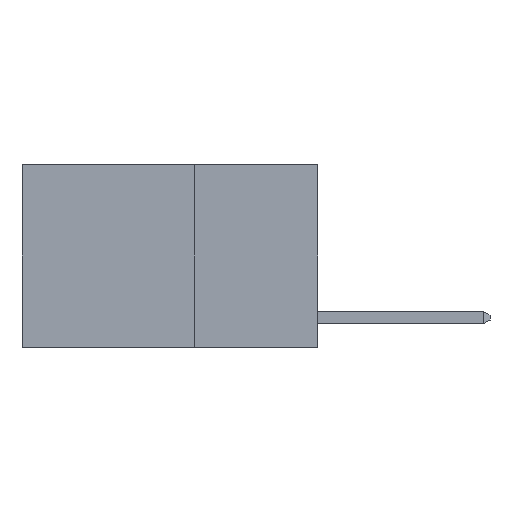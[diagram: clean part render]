
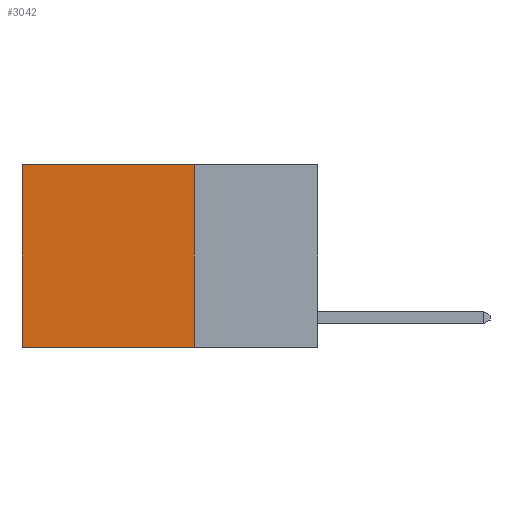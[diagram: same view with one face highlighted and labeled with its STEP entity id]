
A CAD part, left-side view. The second image highlights one B-rep face of the part: STEP entity #3042.
In plain terms, the highlighted planar face has unit normal (-1, 0, 0).
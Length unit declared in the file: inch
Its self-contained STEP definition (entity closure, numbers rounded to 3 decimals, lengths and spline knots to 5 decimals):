
#487 = EDGE_LOOP ( 'NONE', ( #1134, #1333, #1735, #3691 ) ) ;
#552 = CARTESIAN_POINT ( 'NONE',  ( 0.2625, 0.6, 0. ) ) ;
#843 = VECTOR ( 'NONE', #7384, 39.37008 ) ;
#1086 = LINE ( 'NONE', #552, #7396 ) ;
#1132 = VERTEX_POINT ( 'NONE', #3738 ) ;
#1134 = ORIENTED_EDGE ( 'NONE', *, *, #3964, .T. ) ;
#1333 = ORIENTED_EDGE ( 'NONE', *, *, #3685, .F. ) ;
#1570 = VERTEX_POINT ( 'NONE', #8058 ) ;
#1735 = ORIENTED_EDGE ( 'NONE', *, *, #3491, .F. ) ;
#2624 = VECTOR ( 'NONE', #4058, 39.37008 ) ;
#2630 = CARTESIAN_POINT ( 'NONE',  ( 0.2625, 0.25, 0. ) ) ;
#2750 = DIRECTION ( 'NONE',  ( 0., 0., -1. ) ) ;
#3031 = CARTESIAN_POINT ( 'NONE',  ( 0.2625, 0.25, 0. ) ) ;
#3042 = ADVANCED_FACE ( 'NONE', ( #3602 ), #6701, .F. ) ;
#3483 = VECTOR ( 'NONE', #3629, 39.37008 ) ;
#3491 = EDGE_CURVE ( 'NONE', #4470, #3784, #6822, .T. ) ;
#3602 = FACE_OUTER_BOUND ( 'NONE', #487, .T. ) ;
#3629 = DIRECTION ( 'NONE',  ( 0., 0., -1. ) ) ;
#3658 = CARTESIAN_POINT ( 'NONE',  ( 0.2625, 0.25, 0. ) ) ;
#3685 = EDGE_CURVE ( 'NONE', #3784, #1132, #4596, .T. ) ;
#3691 = ORIENTED_EDGE ( 'NONE', *, *, #4253, .T. ) ;
#3738 = CARTESIAN_POINT ( 'NONE',  ( 0.2625, 0.6, -0.37 ) ) ;
#3784 = VERTEX_POINT ( 'NONE', #5549 ) ;
#3964 = EDGE_CURVE ( 'NONE', #1570, #1132, #1086, .T. ) ;
#4058 = DIRECTION ( 'NONE',  ( 0., 1., 0. ) ) ;
#4253 = EDGE_CURVE ( 'NONE', #4470, #1570, #5881, .T. ) ;
#4470 = VERTEX_POINT ( 'NONE', #7191 ) ;
#4556 = DIRECTION ( 'NONE',  ( 0., 0., -1. ) ) ;
#4596 = LINE ( 'NONE', #7111, #2624 ) ;
#5549 = CARTESIAN_POINT ( 'NONE',  ( 0.2625, 0.25, -0.37 ) ) ;
#5643 = AXIS2_PLACEMENT_3D ( 'NONE', #2630, #6667, #2750 ) ;
#5881 = LINE ( 'NONE', #3031, #843 ) ;
#6667 = DIRECTION ( 'NONE',  ( 1., 0., 0. ) ) ;
#6701 = PLANE ( 'NONE',  #5643 ) ;
#6822 = LINE ( 'NONE', #3658, #3483 ) ;
#7111 = CARTESIAN_POINT ( 'NONE',  ( 0.2625, 0.25, -0.37 ) ) ;
#7191 = CARTESIAN_POINT ( 'NONE',  ( 0.2625, 0.25, 0. ) ) ;
#7384 = DIRECTION ( 'NONE',  ( 0., 1., 0. ) ) ;
#7396 = VECTOR ( 'NONE', #4556, 39.37008 ) ;
#8058 = CARTESIAN_POINT ( 'NONE',  ( 0.2625, 0.6, 0. ) ) ;
